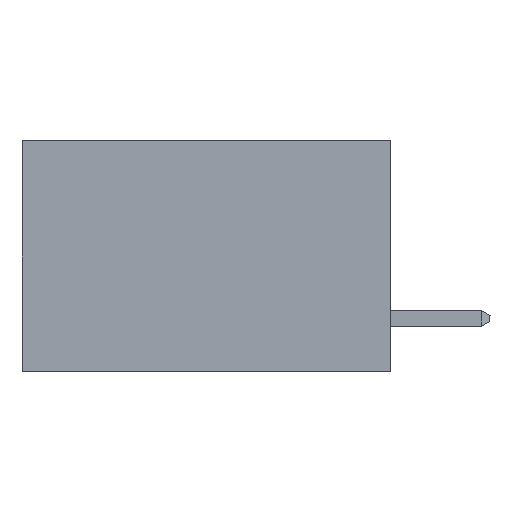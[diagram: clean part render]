
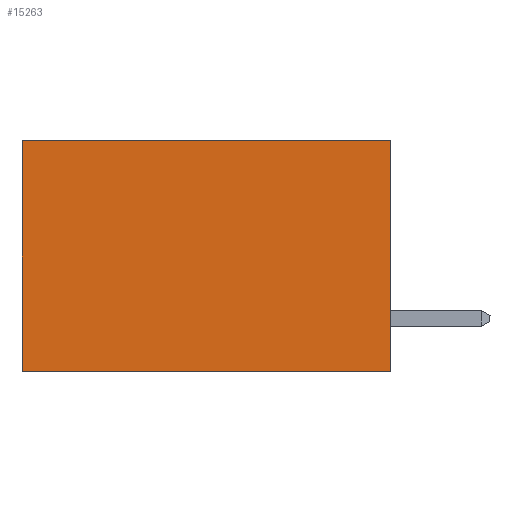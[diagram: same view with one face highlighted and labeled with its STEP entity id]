
A CAD part, left-side view. The second image highlights one B-rep face of the part: STEP entity #15263.
In plain terms, the highlighted planar face has unit normal (-1, 0, 0).
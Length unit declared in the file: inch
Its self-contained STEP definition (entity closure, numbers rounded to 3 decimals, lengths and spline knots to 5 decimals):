
#95 = DIRECTION ( 'NONE',  ( 0., 0., -1. ) ) ;
#216 = ORIENTED_EDGE ( 'NONE', *, *, #3603, .T. ) ;
#488 = DIRECTION ( 'NONE',  ( 1., 0., 0. ) ) ;
#873 = VERTEX_POINT ( 'NONE', #3779 ) ;
#1708 = EDGE_CURVE ( 'NONE', #3269, #18328, #17179, .T. ) ;
#1895 = ORIENTED_EDGE ( 'NONE', *, *, #16187, .F. ) ;
#2680 = VECTOR ( 'NONE', #95, 39.37008 ) ;
#3269 = VERTEX_POINT ( 'NONE', #15953 ) ;
#3443 = VECTOR ( 'NONE', #19352, 39.37008 ) ;
#3603 = EDGE_CURVE ( 'NONE', #18328, #873, #11679, .T. ) ;
#3779 = CARTESIAN_POINT ( 'NONE',  ( 0.277, 0.59, -0.37 ) ) ;
#3862 = CARTESIAN_POINT ( 'NONE',  ( 0.277, 0., -0.37 ) ) ;
#4120 = ORIENTED_EDGE ( 'NONE', *, *, #18127, .F. ) ;
#4897 = VERTEX_POINT ( 'NONE', #3862 ) ;
#4965 = ORIENTED_EDGE ( 'NONE', *, *, #1708, .T. ) ;
#6053 = LINE ( 'NONE', #18605, #14766 ) ;
#7260 = PLANE ( 'NONE',  #14921 ) ;
#11679 = LINE ( 'NONE', #17427, #20150 ) ;
#11843 = EDGE_LOOP ( 'NONE', ( #216, #1895, #4120, #4965 ) ) ;
#12091 = CARTESIAN_POINT ( 'NONE',  ( 0.277, 0., -0.37 ) ) ;
#14766 = VECTOR ( 'NONE', #20162, 39.37008 ) ;
#14921 = AXIS2_PLACEMENT_3D ( 'NONE', #15951, #488, #19286 ) ;
#15263 = ADVANCED_FACE ( 'NONE', ( #16964 ), #7260, .F. ) ;
#15951 = CARTESIAN_POINT ( 'NONE',  ( 0.277, 0., -0.37 ) ) ;
#15953 = CARTESIAN_POINT ( 'NONE',  ( 0.277, 0., 0. ) ) ;
#16187 = EDGE_CURVE ( 'NONE', #4897, #873, #6053, .T. ) ;
#16301 = DIRECTION ( 'NONE',  ( 0., 0., -1. ) ) ;
#16964 = FACE_OUTER_BOUND ( 'NONE', #11843, .T. ) ;
#17179 = LINE ( 'NONE', #19284, #3443 ) ;
#17427 = CARTESIAN_POINT ( 'NONE',  ( 0.277, 0.59, -0.37 ) ) ;
#17725 = CARTESIAN_POINT ( 'NONE',  ( 0.277, 0.59, 0. ) ) ;
#18127 = EDGE_CURVE ( 'NONE', #3269, #4897, #20775, .T. ) ;
#18328 = VERTEX_POINT ( 'NONE', #17725 ) ;
#18605 = CARTESIAN_POINT ( 'NONE',  ( 0.277, 0., -0.37 ) ) ;
#19284 = CARTESIAN_POINT ( 'NONE',  ( 0.277, 0., 0. ) ) ;
#19286 = DIRECTION ( 'NONE',  ( 0., 0., -1. ) ) ;
#19352 = DIRECTION ( 'NONE',  ( 0., 1., 0. ) ) ;
#20150 = VECTOR ( 'NONE', #16301, 39.37008 ) ;
#20162 = DIRECTION ( 'NONE',  ( 0., 1., 0. ) ) ;
#20775 = LINE ( 'NONE', #12091, #2680 ) ;
